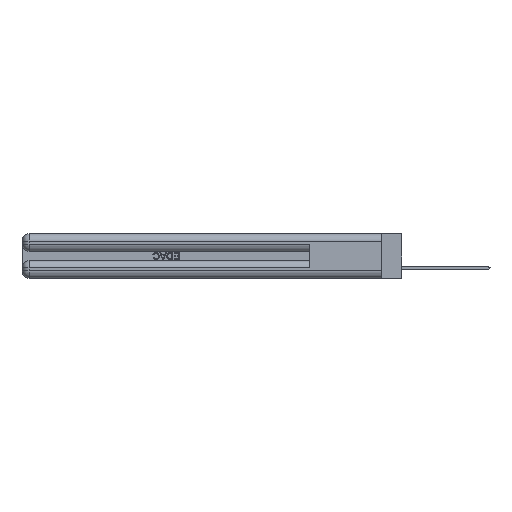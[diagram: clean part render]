
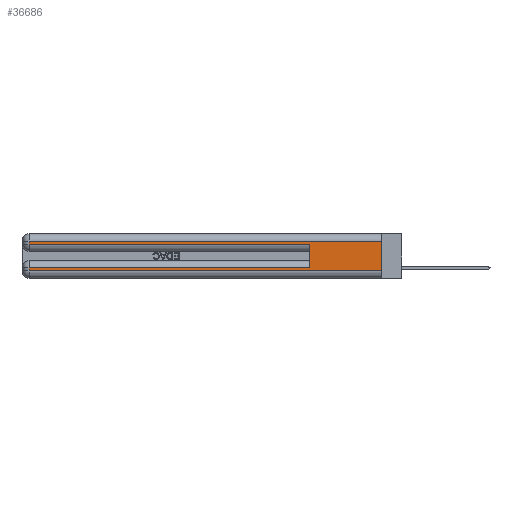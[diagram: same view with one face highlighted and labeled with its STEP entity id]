
A CAD part, left-side view. The second image highlights one B-rep face of the part: STEP entity #36686.
In plain terms, the highlighted planar face has unit normal (-1, 0, 0).
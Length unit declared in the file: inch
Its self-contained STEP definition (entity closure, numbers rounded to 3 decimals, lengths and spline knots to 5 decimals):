
#529 = DIRECTION ( 'NONE',  ( 0., 1., 0. ) ) ;
#1182 = VERTEX_POINT ( 'NONE', #21591 ) ;
#1531 = CARTESIAN_POINT ( 'NONE',  ( 0., 0., 0.37 ) ) ;
#1752 = LINE ( 'NONE', #5654, #28068 ) ;
#3058 = VECTOR ( 'NONE', #12156, 39.37008 ) ;
#5204 = CARTESIAN_POINT ( 'NONE',  ( 0., 2.94, 0.37 ) ) ;
#5654 = CARTESIAN_POINT ( 'NONE',  ( 0., 0., 0.06 ) ) ;
#5936 = ORIENTED_EDGE ( 'NONE', *, *, #38981, .T. ) ;
#8146 = ORIENTED_EDGE ( 'NONE', *, *, #39756, .T. ) ;
#8405 = CARTESIAN_POINT ( 'NONE',  ( 0., 0., 0.31 ) ) ;
#10003 = CARTESIAN_POINT ( 'NONE',  ( 0., 2.94, 0.31 ) ) ;
#10202 = EDGE_CURVE ( 'NONE', #29576, #25830, #38768, .T. ) ;
#10567 = ORIENTED_EDGE ( 'NONE', *, *, #33106, .T. ) ;
#11110 = ORIENTED_EDGE ( 'NONE', *, *, #42833, .T. ) ;
#11921 = LINE ( 'NONE', #15834, #37643 ) ;
#12156 = DIRECTION ( 'NONE',  ( 0., 0., -1. ) ) ;
#12681 = VECTOR ( 'NONE', #40004, 39.37008 ) ;
#13671 = LINE ( 'NONE', #23107, #12681 ) ;
#15075 = LINE ( 'NONE', #39861, #39314 ) ;
#15206 = LINE ( 'NONE', #37603, #29948 ) ;
#15278 = EDGE_CURVE ( 'NONE', #29576, #1182, #11921, .T. ) ;
#15834 = CARTESIAN_POINT ( 'NONE',  ( 0., 0., 0.37 ) ) ;
#18563 = ORIENTED_EDGE ( 'NONE', *, *, #40517, .T. ) ;
#20138 = FACE_OUTER_BOUND ( 'NONE', #41820, .T. ) ;
#21246 = EDGE_CURVE ( 'NONE', #26604, #23313, #36814, .T. ) ;
#21591 = CARTESIAN_POINT ( 'NONE',  ( 0., 0., 0.06 ) ) ;
#21746 = DIRECTION ( 'NONE',  ( 0., 0., 1. ) ) ;
#22566 = DIRECTION ( 'NONE',  ( 0., -1., 0. ) ) ;
#23107 = CARTESIAN_POINT ( 'NONE',  ( 0., 2.94, 0.37 ) ) ;
#23313 = VERTEX_POINT ( 'NONE', #25218 ) ;
#24396 = VERTEX_POINT ( 'NONE', #32806 ) ;
#25218 = CARTESIAN_POINT ( 'NONE',  ( 0., 0.6, 0.285 ) ) ;
#25566 = DIRECTION ( 'NONE',  ( 1., 0., 0. ) ) ;
#25822 = AXIS2_PLACEMENT_3D ( 'NONE', #1531, #25566, #31717 ) ;
#25830 = VERTEX_POINT ( 'NONE', #10003 ) ;
#25947 = CARTESIAN_POINT ( 'NONE',  ( 0., 0.6, 0.085 ) ) ;
#26604 = VERTEX_POINT ( 'NONE', #25947 ) ;
#27340 = ORIENTED_EDGE ( 'NONE', *, *, #15278, .F. ) ;
#27859 = VERTEX_POINT ( 'NONE', #33792 ) ;
#28068 = VECTOR ( 'NONE', #22566, 39.37008 ) ;
#29576 = VERTEX_POINT ( 'NONE', #32928 ) ;
#29728 = DIRECTION ( 'NONE',  ( 0., 1., 0. ) ) ;
#29948 = VECTOR ( 'NONE', #529, 39.37008 ) ;
#30019 = ORIENTED_EDGE ( 'NONE', *, *, #10202, .T. ) ;
#30854 = VECTOR ( 'NONE', #29728, 39.37008 ) ;
#31436 = LINE ( 'NONE', #5204, #3058 ) ;
#31717 = DIRECTION ( 'NONE',  ( 0., 0., -1. ) ) ;
#31939 = ORIENTED_EDGE ( 'NONE', *, *, #21246, .F. ) ;
#32767 = DIRECTION ( 'NONE',  ( 0., 0., -1. ) ) ;
#32806 = CARTESIAN_POINT ( 'NONE',  ( 0., 2.94, 0.085 ) ) ;
#32928 = CARTESIAN_POINT ( 'NONE',  ( 0., 0., 0.31 ) ) ;
#33106 = EDGE_CURVE ( 'NONE', #24396, #38655, #13671, .T. ) ;
#33792 = CARTESIAN_POINT ( 'NONE',  ( 0., 2.94, 0.285 ) ) ;
#35391 = PLANE ( 'NONE',  #25822 ) ;
#35754 = VECTOR ( 'NONE', #21746, 39.37008 ) ;
#36326 = CARTESIAN_POINT ( 'NONE',  ( 0., 2.94, 0.06 ) ) ;
#36686 = ADVANCED_FACE ( 'NONE', ( #20138 ), #35391, .F. ) ;
#36764 = DIRECTION ( 'NONE',  ( 0., -1., 0. ) ) ;
#36814 = LINE ( 'NONE', #41879, #35754 ) ;
#37603 = CARTESIAN_POINT ( 'NONE',  ( 0., 0., 0.085 ) ) ;
#37643 = VECTOR ( 'NONE', #32767, 39.37008 ) ;
#38655 = VERTEX_POINT ( 'NONE', #36326 ) ;
#38768 = LINE ( 'NONE', #8405, #30854 ) ;
#38981 = EDGE_CURVE ( 'NONE', #26604, #24396, #15206, .T. ) ;
#39314 = VECTOR ( 'NONE', #36764, 39.37008 ) ;
#39756 = EDGE_CURVE ( 'NONE', #25830, #27859, #31436, .T. ) ;
#39861 = CARTESIAN_POINT ( 'NONE',  ( 0., 0., 0.285 ) ) ;
#40004 = DIRECTION ( 'NONE',  ( 0., 0., -1. ) ) ;
#40517 = EDGE_CURVE ( 'NONE', #27859, #23313, #15075, .T. ) ;
#41820 = EDGE_LOOP ( 'NONE', ( #27340, #30019, #8146, #18563, #31939, #5936, #10567, #11110 ) ) ;
#41879 = CARTESIAN_POINT ( 'NONE',  ( 0., 0.6, 0.145 ) ) ;
#42833 = EDGE_CURVE ( 'NONE', #38655, #1182, #1752, .T. ) ;
